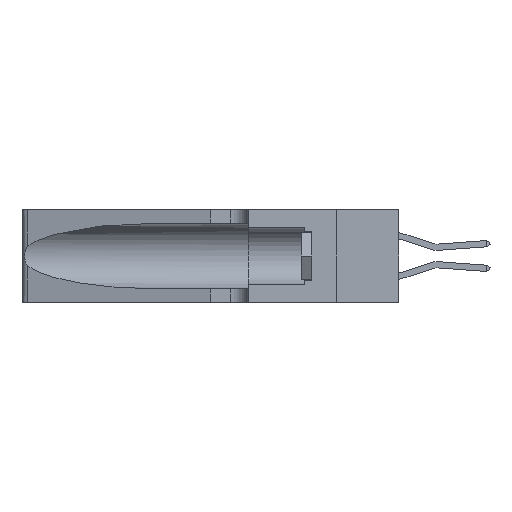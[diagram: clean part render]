
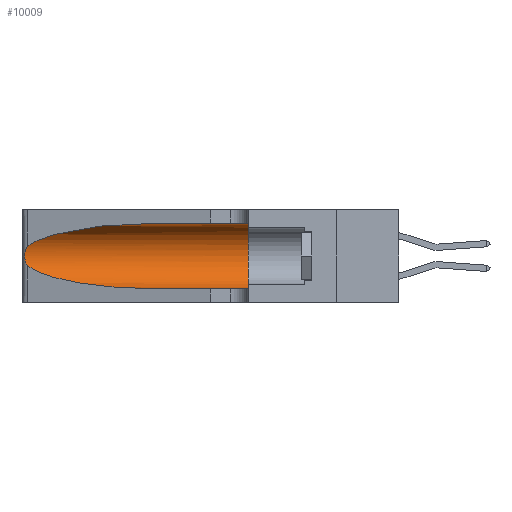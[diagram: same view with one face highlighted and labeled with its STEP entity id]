
A CAD part, left-side view. The second image highlights one B-rep face of the part: STEP entity #10009.
In plain terms, the highlighted cylindrical face has radius 3.308 mm (diameter 6.617 mm), a partial arc.
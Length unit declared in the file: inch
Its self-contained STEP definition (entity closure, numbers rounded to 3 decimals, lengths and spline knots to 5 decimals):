
#72 = EDGE_CURVE ( 'NONE', #19057, #22084, #2389, .T. ) ;
#510 = B_SPLINE_CURVE_WITH_KNOTS ( 'NONE', 3,
 ( #15857, #778, #17708, #6569, #19564, #8476, #21378, #10344, #23216, #12239, #865, #14076, #2808, #15933 ),
 .UNSPECIFIED., .F., .F.,
 ( 4, 2, 2, 2, 2, 2, 4 ),
 ( 0., 0.00027, 0.00053, 0.00107, 0.0016, 0.00187, 0.00214 ),
 .UNSPECIFIED. ) ;
#743 = CARTESIAN_POINT ( 'NONE',  ( 0.1305, 0.72297, 0.31525 ) ) ;
#778 = CARTESIAN_POINT ( 'NONE',  ( 0.25555, 1.22994, 0.2215 ) ) ;
#865 = CARTESIAN_POINT ( 'NONE',  ( 0.25789, 1.23486, 0.15765 ) ) ;
#983 =( BOUNDED_CURVE ( )  B_SPLINE_CURVE ( 3, ( #10673, #16261, #21774, #10755 ),
 .UNSPECIFIED., .F., .T. ) 
 B_SPLINE_CURVE_WITH_KNOTS ( ( 4, 4 ),
 ( 1.5708, 2.84003 ),
 .UNSPECIFIED. ) 
 CURVE ( )  GEOMETRIC_REPRESENTATION_ITEM ( )  RATIONAL_B_SPLINE_CURVE ( ( 1., 0.87, 0.87, 1. ) ) 
 REPRESENTATION_ITEM ( '' )  );
#1756 = CARTESIAN_POINT ( 'NONE',  ( 0.25487, 1.22718, 0.14631 ) ) ;
#2283 = CARTESIAN_POINT ( 'NONE',  ( 0.2373, 1.15595, 0.08982 ) ) ;
#2389 =( BOUNDED_CURVE ( )  B_SPLINE_CURVE ( 3, ( #1756, #2283, #3497, #3444 ),
 .UNSPECIFIED., .F., .F. ) 
 B_SPLINE_CURVE_WITH_KNOTS ( ( 4, 4 ),
 ( 3.44316, 4.71239 ),
 .UNSPECIFIED. ) 
 CURVE ( )  GEOMETRIC_REPRESENTATION_ITEM ( )  RATIONAL_B_SPLINE_CURVE ( ( 1., 0.87, 0.87, 1. ) ) 
 REPRESENTATION_ITEM ( '' )  );
#2407 = CARTESIAN_POINT ( 'NONE',  ( 0.1305, 0.35, 0.05475 ) ) ;
#2808 = CARTESIAN_POINT ( 'NONE',  ( 0.25555, 1.22993, 0.14849 ) ) ;
#2876 = VECTOR ( 'NONE', #21488, 39.37008 ) ;
#2889 = CIRCLE ( 'NONE', #5568, 0.13025 ) ;
#2928 = AXIS2_PLACEMENT_3D ( 'NONE', #7686, #9592, #3880 ) ;
#3444 = CARTESIAN_POINT ( 'NONE',  ( 0.1305, 0.72297, 0.05475 ) ) ;
#3497 = CARTESIAN_POINT ( 'NONE',  ( 0.18966, 0.96281, 0.05475 ) ) ;
#3880 = DIRECTION ( 'NONE',  ( 0., 0., -1. ) ) ;
#4200 = ORIENTED_EDGE ( 'NONE', *, *, #13706, .T. ) ;
#4933 = ORIENTED_EDGE ( 'NONE', *, *, #9643, .T. ) ;
#5368 = EDGE_CURVE ( 'NONE', #20675, #8952, #17251, .T. ) ;
#5568 = AXIS2_PLACEMENT_3D ( 'NONE', #11270, #24097, #13129 ) ;
#5851 = VERTEX_POINT ( 'NONE', #2407 ) ;
#6569 = CARTESIAN_POINT ( 'NONE',  ( 0.25787, 1.23484, 0.2124 ) ) ;
#7686 = CARTESIAN_POINT ( 'NONE',  ( 0.1305, 1.61858, 0.185 ) ) ;
#8340 = CARTESIAN_POINT ( 'NONE',  ( 0.1305, 0.72297, 0.05475 ) ) ;
#8476 = CARTESIAN_POINT ( 'NONE',  ( 0.26018, 1.23835, 0.19895 ) ) ;
#8952 = VERTEX_POINT ( 'NONE', #21483 ) ;
#8981 = VERTEX_POINT ( 'NONE', #17894 ) ;
#9592 = DIRECTION ( 'NONE',  ( 0., -1., 0. ) ) ;
#9643 = EDGE_CURVE ( 'NONE', #20675, #8981, #983, .T. ) ;
#10009 = ADVANCED_FACE ( 'NONE', ( #18470 ), #13878, .F. ) ;
#10344 = CARTESIAN_POINT ( 'NONE',  ( 0.26075, 1.23896, 0.178 ) ) ;
#10457 = CARTESIAN_POINT ( 'NONE',  ( 0.1305, 1.61858, 0.31525 ) ) ;
#10673 = CARTESIAN_POINT ( 'NONE',  ( 0.1305, 0.72297, 0.31525 ) ) ;
#10755 = CARTESIAN_POINT ( 'NONE',  ( 0.25487, 1.22718, 0.22369 ) ) ;
#11270 = CARTESIAN_POINT ( 'NONE',  ( 0.1305, 0.35, 0.185 ) ) ;
#12239 = CARTESIAN_POINT ( 'NONE',  ( 0.25856, 1.23593, 0.16098 ) ) ;
#13039 = VECTOR ( 'NONE', #13197, 39.37008 ) ;
#13129 = DIRECTION ( 'NONE',  ( 0., 0., 1. ) ) ;
#13197 = DIRECTION ( 'NONE',  ( 0., -1., 0. ) ) ;
#13706 = EDGE_CURVE ( 'NONE', #8981, #19057, #510, .T. ) ;
#13878 = CYLINDRICAL_SURFACE ( 'NONE', #2928, 0.13025 ) ;
#14076 = CARTESIAN_POINT ( 'NONE',  ( 0.25639, 1.23186, 0.15144 ) ) ;
#14961 = CARTESIAN_POINT ( 'NONE',  ( 0.1305, 1.61858, 0.05475 ) ) ;
#15396 = EDGE_CURVE ( 'NONE', #8952, #5851, #2889, .T. ) ;
#15857 = CARTESIAN_POINT ( 'NONE',  ( 0.25487, 1.22718, 0.22369 ) ) ;
#15933 = CARTESIAN_POINT ( 'NONE',  ( 0.25487, 1.22718, 0.14631 ) ) ;
#16261 = CARTESIAN_POINT ( 'NONE',  ( 0.18966, 0.96281, 0.31525 ) ) ;
#17251 = LINE ( 'NONE', #10457, #2876 ) ;
#17708 = CARTESIAN_POINT ( 'NONE',  ( 0.25639, 1.23184, 0.21858 ) ) ;
#17894 = CARTESIAN_POINT ( 'NONE',  ( 0.25487, 1.22718, 0.22369 ) ) ;
#17936 = LINE ( 'NONE', #14961, #13039 ) ;
#18470 = FACE_OUTER_BOUND ( 'NONE', #22294, .T. ) ;
#19057 = VERTEX_POINT ( 'NONE', #20547 ) ;
#19564 = CARTESIAN_POINT ( 'NONE',  ( 0.25854, 1.2359, 0.20912 ) ) ;
#19583 = ORIENTED_EDGE ( 'NONE', *, *, #72, .T. ) ;
#20547 = CARTESIAN_POINT ( 'NONE',  ( 0.25487, 1.22718, 0.14631 ) ) ;
#20675 = VERTEX_POINT ( 'NONE', #743 ) ;
#20742 = ORIENTED_EDGE ( 'NONE', *, *, #5368, .F. ) ;
#21378 = CARTESIAN_POINT ( 'NONE',  ( 0.26075, 1.23896, 0.19203 ) ) ;
#21483 = CARTESIAN_POINT ( 'NONE',  ( 0.1305, 0.35, 0.31525 ) ) ;
#21488 = DIRECTION ( 'NONE',  ( 0., -1., 0. ) ) ;
#21774 = CARTESIAN_POINT ( 'NONE',  ( 0.2373, 1.15595, 0.28018 ) ) ;
#22084 = VERTEX_POINT ( 'NONE', #8340 ) ;
#22294 = EDGE_LOOP ( 'NONE', ( #4933, #4200, #19583, #23177, #22902, #20742 ) ) ;
#22902 = ORIENTED_EDGE ( 'NONE', *, *, #15396, .F. ) ;
#23027 = EDGE_CURVE ( 'NONE', #22084, #5851, #17936, .T. ) ;
#23177 = ORIENTED_EDGE ( 'NONE', *, *, #23027, .T. ) ;
#23216 = CARTESIAN_POINT ( 'NONE',  ( 0.26017, 1.23833, 0.17102 ) ) ;
#24097 = DIRECTION ( 'NONE',  ( 0., 1., 0. ) ) ;
